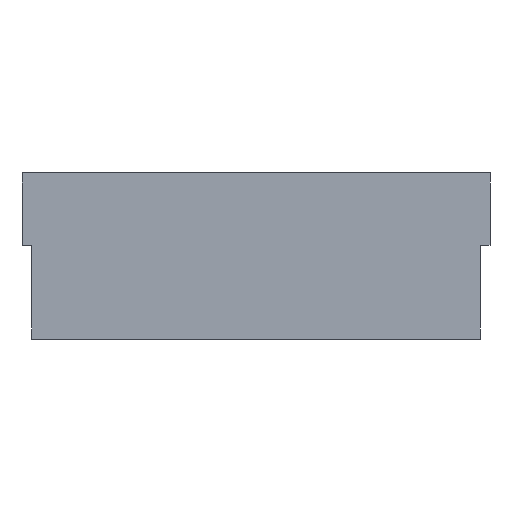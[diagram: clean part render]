
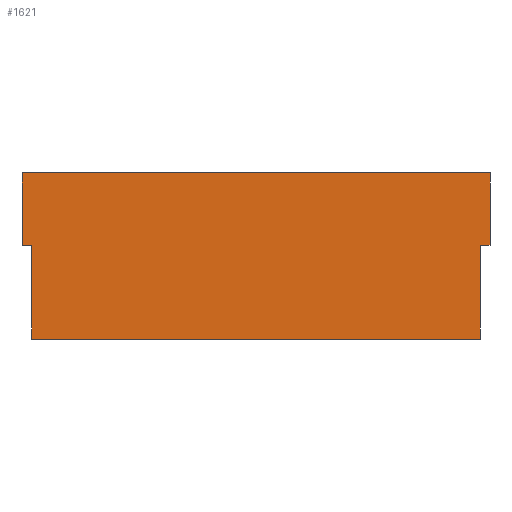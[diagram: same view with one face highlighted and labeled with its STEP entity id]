
A CAD part, front view. The second image highlights one B-rep face of the part: STEP entity #1621.
In plain terms, the highlighted planar face has unit normal (0, -1, 0).
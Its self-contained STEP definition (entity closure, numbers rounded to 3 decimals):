
#9 = ORIENTED_EDGE ( 'NONE', *, *, #1281, .T. ) ;
#104 = VERTEX_POINT ( 'NONE', #262 ) ;
#262 = CARTESIAN_POINT ( 'NONE',  ( 20., -3.15, 7.1 ) ) ;
#641 = EDGE_CURVE ( 'NONE', #1730, #9328, #12804, .T. ) ;
#666 = VERTEX_POINT ( 'NONE', #8455 ) ;
#1097 = DIRECTION ( 'NONE',  ( 0., 0., -1. ) ) ;
#1221 = CARTESIAN_POINT ( 'NONE',  ( 20., -3.15, 0.9 ) ) ;
#1259 = AXIS2_PLACEMENT_3D ( 'NONE', #6931, #3635, #10795 ) ;
#1281 = EDGE_CURVE ( 'NONE', #11986, #666, #10816, .T. ) ;
#1391 = ORIENTED_EDGE ( 'NONE', *, *, #641, .T. ) ;
#1472 = VECTOR ( 'NONE', #1097, 1000. ) ;
#1621 = ADVANCED_FACE ( 'NONE', ( #2601 ), #5481, .F. ) ;
#1715 = EDGE_CURVE ( 'NONE', #9709, #8924, #10493, .T. ) ;
#1730 = VERTEX_POINT ( 'NONE', #7074 ) ;
#2483 = LINE ( 'NONE', #11875, #12579 ) ;
#2601 = FACE_OUTER_BOUND ( 'NONE', #6095, .T. ) ;
#3176 = LINE ( 'NONE', #10741, #5877 ) ;
#3315 = CARTESIAN_POINT ( 'NONE',  ( -19.15, -3.15, 0.9 ) ) ;
#3413 = CARTESIAN_POINT ( 'NONE',  ( 20., -3.15, 7.1 ) ) ;
#3635 = DIRECTION ( 'NONE',  ( 0., 1., 0. ) ) ;
#3968 = ORIENTED_EDGE ( 'NONE', *, *, #6044, .T. ) ;
#4090 = VECTOR ( 'NONE', #5286, 1000. ) ;
#4534 = LINE ( 'NONE', #13095, #13312 ) ;
#5110 = CARTESIAN_POINT ( 'NONE',  ( 19.15, -3.15, 0.9 ) ) ;
#5286 = DIRECTION ( 'NONE',  ( 1., 0., 0. ) ) ;
#5442 = CARTESIAN_POINT ( 'NONE',  ( -20., -3.15, 7.1 ) ) ;
#5481 = PLANE ( 'NONE',  #1259 ) ;
#5500 = DIRECTION ( 'NONE',  ( 1., 0., 0. ) ) ;
#5654 = LINE ( 'NONE', #3413, #8620 ) ;
#5877 = VECTOR ( 'NONE', #9620, 1000. ) ;
#6044 = EDGE_CURVE ( 'NONE', #9995, #8924, #4534, .T. ) ;
#6095 = EDGE_LOOP ( 'NONE', ( #10145, #11937, #9, #7178, #13193, #1391, #7001, #3968 ) ) ;
#6169 = CARTESIAN_POINT ( 'NONE',  ( -20., -3.15, 0.9 ) ) ;
#6773 = DIRECTION ( 'NONE',  ( 0., 0., -1. ) ) ;
#6931 = CARTESIAN_POINT ( 'NONE',  ( 20., -3.15, 7.1 ) ) ;
#7001 = ORIENTED_EDGE ( 'NONE', *, *, #10164, .T. ) ;
#7074 = CARTESIAN_POINT ( 'NONE',  ( -20., -3.15, 7.1 ) ) ;
#7178 = ORIENTED_EDGE ( 'NONE', *, *, #12494, .F. ) ;
#7277 = DIRECTION ( 'NONE',  ( -1., 0., 0. ) ) ;
#7433 = LINE ( 'NONE', #3315, #4090 ) ;
#7890 = DIRECTION ( 'NONE',  ( -1., 0., 0. ) ) ;
#8368 = EDGE_CURVE ( 'NONE', #104, #1730, #5654, .T. ) ;
#8418 = VECTOR ( 'NONE', #5500, 1000. ) ;
#8455 = CARTESIAN_POINT ( 'NONE',  ( 20., -3.15, 0.9 ) ) ;
#8615 = VECTOR ( 'NONE', #7277, 1000. ) ;
#8620 = VECTOR ( 'NONE', #7890, 1000. ) ;
#8924 = VERTEX_POINT ( 'NONE', #10383 ) ;
#9328 = VERTEX_POINT ( 'NONE', #6169 ) ;
#9620 = DIRECTION ( 'NONE',  ( 0., 0., -1. ) ) ;
#9699 = DIRECTION ( 'NONE',  ( 0., 0., -1. ) ) ;
#9709 = VERTEX_POINT ( 'NONE', #13586 ) ;
#9995 = VERTEX_POINT ( 'NONE', #13079 ) ;
#10145 = ORIENTED_EDGE ( 'NONE', *, *, #1715, .F. ) ;
#10164 = EDGE_CURVE ( 'NONE', #9328, #9995, #7433, .T. ) ;
#10383 = CARTESIAN_POINT ( 'NONE',  ( -19.15, -3.15, -7.1 ) ) ;
#10493 = LINE ( 'NONE', #11486, #8615 ) ;
#10741 = CARTESIAN_POINT ( 'NONE',  ( 20., -3.15, 7.1 ) ) ;
#10795 = DIRECTION ( 'NONE',  ( 0., 0., 1. ) ) ;
#10816 = LINE ( 'NONE', #1221, #8418 ) ;
#11486 = CARTESIAN_POINT ( 'NONE',  ( 20., -3.15, -7.1 ) ) ;
#11875 = CARTESIAN_POINT ( 'NONE',  ( 19.15, -3.15, 47.593 ) ) ;
#11937 = ORIENTED_EDGE ( 'NONE', *, *, #13629, .F. ) ;
#11986 = VERTEX_POINT ( 'NONE', #5110 ) ;
#12494 = EDGE_CURVE ( 'NONE', #104, #666, #3176, .T. ) ;
#12579 = VECTOR ( 'NONE', #9699, 1000. ) ;
#12804 = LINE ( 'NONE', #5442, #1472 ) ;
#13079 = CARTESIAN_POINT ( 'NONE',  ( -19.15, -3.15, 0.9 ) ) ;
#13095 = CARTESIAN_POINT ( 'NONE',  ( -19.15, -3.15, 47.593 ) ) ;
#13193 = ORIENTED_EDGE ( 'NONE', *, *, #8368, .T. ) ;
#13312 = VECTOR ( 'NONE', #6773, 1000. ) ;
#13586 = CARTESIAN_POINT ( 'NONE',  ( 19.15, -3.15, -7.1 ) ) ;
#13629 = EDGE_CURVE ( 'NONE', #11986, #9709, #2483, .T. ) ;
